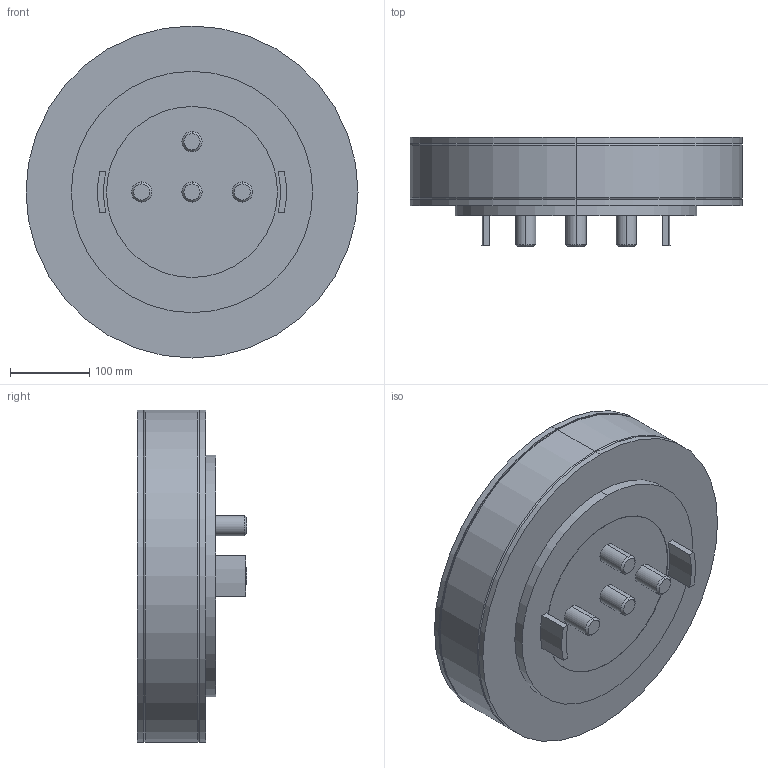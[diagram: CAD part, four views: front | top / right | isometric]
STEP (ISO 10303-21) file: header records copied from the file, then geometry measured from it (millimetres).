
FILE_DESCRIPTION (( 'STEP AP203' ), '1' );
FILE_NAME ('686N05222001G1E.STEP', '2023-04-28T10:48:35', ( '' ), ( '' ), 'SwSTEP 2.0', 'SolidWorks 2020', '' );
FILE_SCHEMA (( 'CONFIG_CONTROL_DESIGN' ));
Length unit declared in the file: inch
Products named in the file (1): 686N05222001G1E
Bounding box: 419.1 x 138.43 x 419.1 mm (x, y, z)
Volume: 12651196.6 mm3; surface area: 435250.5 mm2
Topology: 1 solids, 1 shells, 65 faces, 132 edges, 84 vertices
Faces by surface type: cylinder 24, plane 21, cone 16, torus 4
Entity records: 1809 total; most frequent: DIRECTION 344, CARTESIAN_POINT 282, ORIENTED_EDGE 264, AXIS2_PLACEMENT_3D 146, EDGE_CURVE 132, VERTEX_POINT 84, EDGE_LOOP 80, CIRCLE 80
